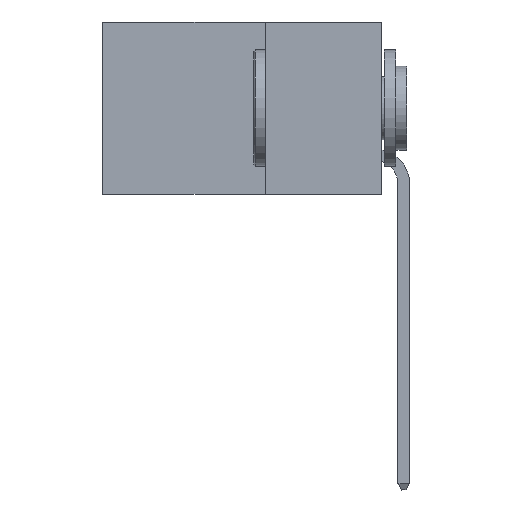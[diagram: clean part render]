
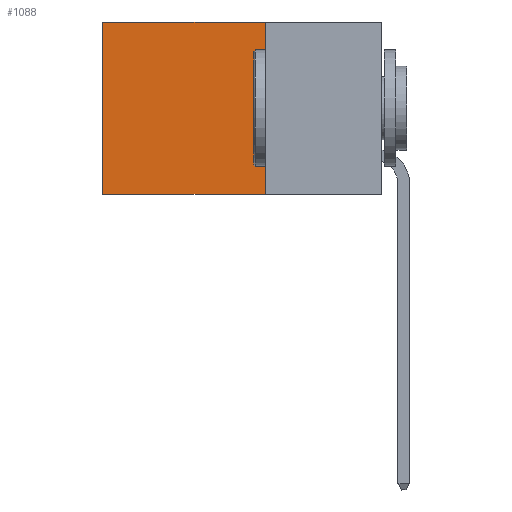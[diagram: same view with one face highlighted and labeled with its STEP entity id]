
A CAD part, left-side view. The second image highlights one B-rep face of the part: STEP entity #1088.
In plain terms, the highlighted planar face has unit normal (-1, 0, 0).
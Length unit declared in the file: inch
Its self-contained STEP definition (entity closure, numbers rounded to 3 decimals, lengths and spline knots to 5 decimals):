
#262 = CARTESIAN_POINT ( 'NONE',  ( 0.2875, 0.6, 0. ) ) ;
#1009 = CARTESIAN_POINT ( 'NONE',  ( 0.2875, 0.25, 0. ) ) ;
#1078 = EDGE_CURVE ( 'NONE', #10415, #7902, #4546, .T. ) ;
#1088 = ADVANCED_FACE ( 'NONE', ( #4165 ), #9219, .F. ) ;
#2451 = CARTESIAN_POINT ( 'NONE',  ( 0.2875, 0.6, -0.37 ) ) ;
#2776 = ORIENTED_EDGE ( 'NONE', *, *, #1078, .F. ) ;
#2799 = LINE ( 'NONE', #262, #7433 ) ;
#2830 = AXIS2_PLACEMENT_3D ( 'NONE', #6648, #4303, #5863 ) ;
#2879 = DIRECTION ( 'NONE',  ( 0., 1., 0. ) ) ;
#3052 = EDGE_CURVE ( 'NONE', #7902, #6991, #10044, .T. ) ;
#4165 = FACE_OUTER_BOUND ( 'NONE', #6559, .T. ) ;
#4194 = LINE ( 'NONE', #8596, #9989 ) ;
#4303 = DIRECTION ( 'NONE',  ( 1., 0., 0. ) ) ;
#4320 = DIRECTION ( 'NONE',  ( 0., 0., -1. ) ) ;
#4546 = LINE ( 'NONE', #6614, #6476 ) ;
#5490 = EDGE_CURVE ( 'NONE', #10415, #10153, #4194, .T. ) ;
#5863 = DIRECTION ( 'NONE',  ( 0., 0., -1. ) ) ;
#6476 = VECTOR ( 'NONE', #9062, 39.37008 ) ;
#6559 = EDGE_LOOP ( 'NONE', ( #9949, #8909, #2776, #9844 ) ) ;
#6614 = CARTESIAN_POINT ( 'NONE',  ( 0.2875, 0.25, 0. ) ) ;
#6648 = CARTESIAN_POINT ( 'NONE',  ( 0.2875, 0.25, 0. ) ) ;
#6826 = VECTOR ( 'NONE', #8766, 39.37008 ) ;
#6991 = VERTEX_POINT ( 'NONE', #2451 ) ;
#7433 = VECTOR ( 'NONE', #4320, 39.37008 ) ;
#7902 = VERTEX_POINT ( 'NONE', #8570 ) ;
#8542 = EDGE_CURVE ( 'NONE', #10153, #6991, #2799, .T. ) ;
#8570 = CARTESIAN_POINT ( 'NONE',  ( 0.2875, 0.25, -0.37 ) ) ;
#8596 = CARTESIAN_POINT ( 'NONE',  ( 0.2875, 0.25, 0. ) ) ;
#8766 = DIRECTION ( 'NONE',  ( 0., 1., 0. ) ) ;
#8909 = ORIENTED_EDGE ( 'NONE', *, *, #3052, .F. ) ;
#9062 = DIRECTION ( 'NONE',  ( 0., 0., -1. ) ) ;
#9219 = PLANE ( 'NONE',  #2830 ) ;
#9844 = ORIENTED_EDGE ( 'NONE', *, *, #5490, .T. ) ;
#9949 = ORIENTED_EDGE ( 'NONE', *, *, #8542, .T. ) ;
#9989 = VECTOR ( 'NONE', #2879, 39.37008 ) ;
#10044 = LINE ( 'NONE', #10419, #6826 ) ;
#10153 = VERTEX_POINT ( 'NONE', #10185 ) ;
#10185 = CARTESIAN_POINT ( 'NONE',  ( 0.2875, 0.6, 0. ) ) ;
#10415 = VERTEX_POINT ( 'NONE', #1009 ) ;
#10419 = CARTESIAN_POINT ( 'NONE',  ( 0.2875, 0.25, -0.37 ) ) ;
